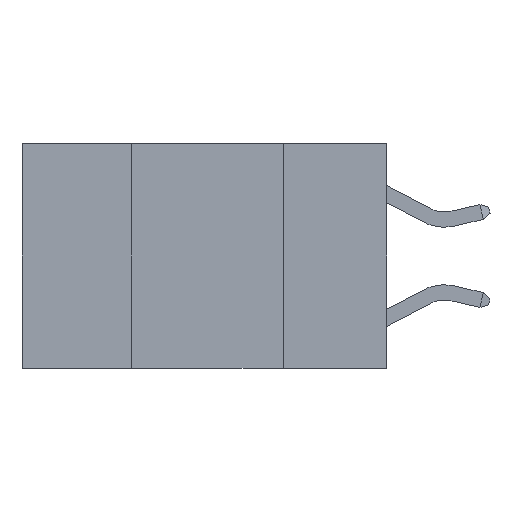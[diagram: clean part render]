
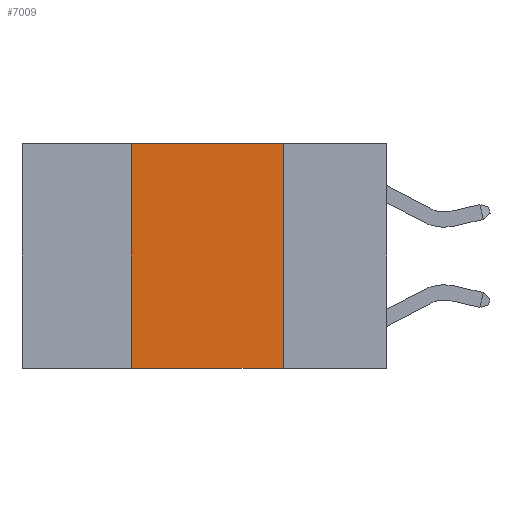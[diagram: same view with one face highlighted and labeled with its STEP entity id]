
A CAD part, left-side view. The second image highlights one B-rep face of the part: STEP entity #7009.
In plain terms, the highlighted planar face has unit normal (-1, 0, 0).
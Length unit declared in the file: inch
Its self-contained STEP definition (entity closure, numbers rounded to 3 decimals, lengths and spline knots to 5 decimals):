
#402 = DIRECTION ( 'NONE',  ( 0., 0., -1. ) ) ;
#1163 = ORIENTED_EDGE ( 'NONE', *, *, #13461, .T. ) ;
#1516 = DIRECTION ( 'NONE',  ( 0., 0., -1. ) ) ;
#1671 = DIRECTION ( 'NONE',  ( 0., -1., 0. ) ) ;
#2446 = LINE ( 'NONE', #23635, #21390 ) ;
#3061 = VERTEX_POINT ( 'NONE', #16590 ) ;
#3279 = AXIS2_PLACEMENT_3D ( 'NONE', #22420, #11461, #402 ) ;
#3571 = EDGE_CURVE ( 'NONE', #13723, #15625, #13616, .T. ) ;
#4879 = ORIENTED_EDGE ( 'NONE', *, *, #3571, .F. ) ;
#5284 = CARTESIAN_POINT ( 'NONE',  ( 0., 0.6, -0.37 ) ) ;
#6043 = EDGE_CURVE ( 'NONE', #9142, #3061, #18368, .T. ) ;
#7009 = ADVANCED_FACE ( 'NONE', ( #12886 ), #7730, .F. ) ;
#7071 = VECTOR ( 'NONE', #7136, 39.37008 ) ;
#7136 = DIRECTION ( 'NONE',  ( 0., -1., 0. ) ) ;
#7730 = PLANE ( 'NONE',  #3279 ) ;
#8655 = VECTOR ( 'NONE', #1516, 39.37008 ) ;
#8769 = VECTOR ( 'NONE', #21683, 39.37008 ) ;
#9142 = VERTEX_POINT ( 'NONE', #23409 ) ;
#11461 = DIRECTION ( 'NONE',  ( 1., 0., 0. ) ) ;
#11999 = LINE ( 'NONE', #5284, #7071 ) ;
#12545 = CARTESIAN_POINT ( 'NONE',  ( 0., 0.17, 0. ) ) ;
#12886 = FACE_OUTER_BOUND ( 'NONE', #16474, .T. ) ;
#13461 = EDGE_CURVE ( 'NONE', #13723, #3061, #11999, .T. ) ;
#13538 = ORIENTED_EDGE ( 'NONE', *, *, #20193, .F. ) ;
#13616 = LINE ( 'NONE', #19845, #8769 ) ;
#13723 = VERTEX_POINT ( 'NONE', #16940 ) ;
#15625 = VERTEX_POINT ( 'NONE', #16107 ) ;
#16107 = CARTESIAN_POINT ( 'NONE',  ( 0., 0.42, 0. ) ) ;
#16474 = EDGE_LOOP ( 'NONE', ( #17256, #13538, #4879, #1163 ) ) ;
#16590 = CARTESIAN_POINT ( 'NONE',  ( 0., 0.17, -0.37 ) ) ;
#16940 = CARTESIAN_POINT ( 'NONE',  ( 0., 0.42, -0.37 ) ) ;
#17256 = ORIENTED_EDGE ( 'NONE', *, *, #6043, .F. ) ;
#18368 = LINE ( 'NONE', #12545, #8655 ) ;
#19845 = CARTESIAN_POINT ( 'NONE',  ( 0., 0.42, 0. ) ) ;
#20193 = EDGE_CURVE ( 'NONE', #15625, #9142, #2446, .T. ) ;
#21390 = VECTOR ( 'NONE', #1671, 39.37008 ) ;
#21683 = DIRECTION ( 'NONE',  ( 0., 0., 1. ) ) ;
#22420 = CARTESIAN_POINT ( 'NONE',  ( 0., 0.6, 0. ) ) ;
#23409 = CARTESIAN_POINT ( 'NONE',  ( 0., 0.17, 0. ) ) ;
#23635 = CARTESIAN_POINT ( 'NONE',  ( 0., 0.6, 0. ) ) ;
